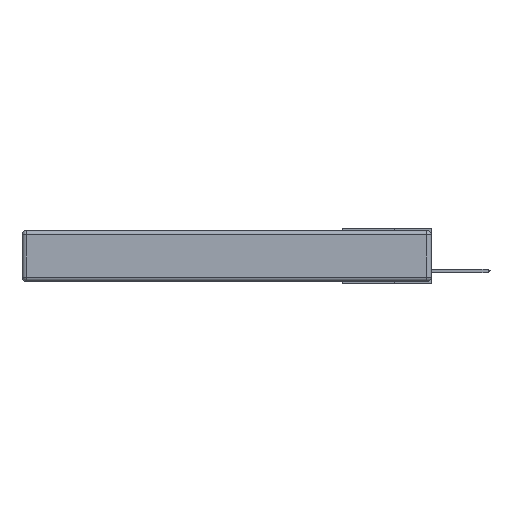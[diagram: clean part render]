
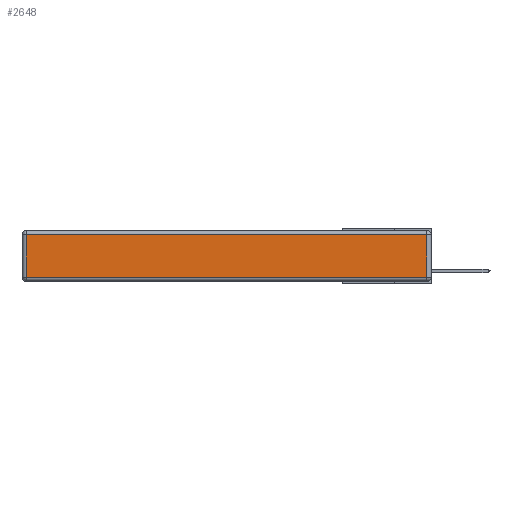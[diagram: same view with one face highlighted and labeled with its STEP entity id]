
A CAD part, left-side view. The second image highlights one B-rep face of the part: STEP entity #2648.
In plain terms, the highlighted planar face has unit normal (-1, 0, 0).
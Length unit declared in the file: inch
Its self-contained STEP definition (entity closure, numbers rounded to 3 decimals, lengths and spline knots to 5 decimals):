
#318 = VERTEX_POINT ( 'NONE', #960 ) ;
#879 = VECTOR ( 'NONE', #4950, 39.37008 ) ;
#960 = CARTESIAN_POINT ( 'NONE',  ( 0., 0.03, -0.03 ) ) ;
#1116 = CARTESIAN_POINT ( 'NONE',  ( 0., 0.03, -0.313 ) ) ;
#1680 = CARTESIAN_POINT ( 'NONE',  ( 0., 0., -0.343 ) ) ;
#1744 = VECTOR ( 'NONE', #12640, 39.37008 ) ;
#2648 = ADVANCED_FACE ( 'NONE', ( #12235 ), #5894, .T. ) ;
#2721 = CARTESIAN_POINT ( 'NONE',  ( 0., 2.72, -0.03 ) ) ;
#2850 = DIRECTION ( 'NONE',  ( 0., 0., 1. ) ) ;
#4533 = EDGE_CURVE ( 'NONE', #13533, #318, #12100, .T. ) ;
#4950 = DIRECTION ( 'NONE',  ( 0., 0., -1. ) ) ;
#5166 = VECTOR ( 'NONE', #6782, 39.37008 ) ;
#5361 = EDGE_CURVE ( 'NONE', #10199, #13533, #7965, .T. ) ;
#5615 = ORIENTED_EDGE ( 'NONE', *, *, #5361, .T. ) ;
#5800 = DIRECTION ( 'NONE',  ( 0., 0., 1. ) ) ;
#5894 = PLANE ( 'NONE',  #9073 ) ;
#6782 = DIRECTION ( 'NONE',  ( 0., -1., 0. ) ) ;
#6821 = EDGE_LOOP ( 'NONE', ( #5615, #12985, #11970, #10059 ) ) ;
#7507 = CARTESIAN_POINT ( 'NONE',  ( 0., 2.75, -0.03 ) ) ;
#7965 = LINE ( 'NONE', #8874, #5166 ) ;
#8053 = CARTESIAN_POINT ( 'NONE',  ( 0., 2.72, -0.343 ) ) ;
#8874 = CARTESIAN_POINT ( 'NONE',  ( 0., 0., -0.313 ) ) ;
#9073 = AXIS2_PLACEMENT_3D ( 'NONE', #1680, #10172, #5800 ) ;
#9204 = CARTESIAN_POINT ( 'NONE',  ( 0., 0.03, -0.343 ) ) ;
#9989 = VECTOR ( 'NONE', #2850, 39.37008 ) ;
#10059 = ORIENTED_EDGE ( 'NONE', *, *, #13163, .T. ) ;
#10125 = CARTESIAN_POINT ( 'NONE',  ( 0., 2.72, -0.313 ) ) ;
#10172 = DIRECTION ( 'NONE',  ( -1., 0., 0. ) ) ;
#10199 = VERTEX_POINT ( 'NONE', #10125 ) ;
#10277 = VERTEX_POINT ( 'NONE', #2721 ) ;
#11858 = EDGE_CURVE ( 'NONE', #318, #10277, #13035, .T. ) ;
#11970 = ORIENTED_EDGE ( 'NONE', *, *, #11858, .T. ) ;
#12100 = LINE ( 'NONE', #9204, #9989 ) ;
#12235 = FACE_OUTER_BOUND ( 'NONE', #6821, .T. ) ;
#12640 = DIRECTION ( 'NONE',  ( 0., 1., 0. ) ) ;
#12839 = LINE ( 'NONE', #8053, #879 ) ;
#12985 = ORIENTED_EDGE ( 'NONE', *, *, #4533, .T. ) ;
#13035 = LINE ( 'NONE', #7507, #1744 ) ;
#13163 = EDGE_CURVE ( 'NONE', #10277, #10199, #12839, .T. ) ;
#13533 = VERTEX_POINT ( 'NONE', #1116 ) ;
